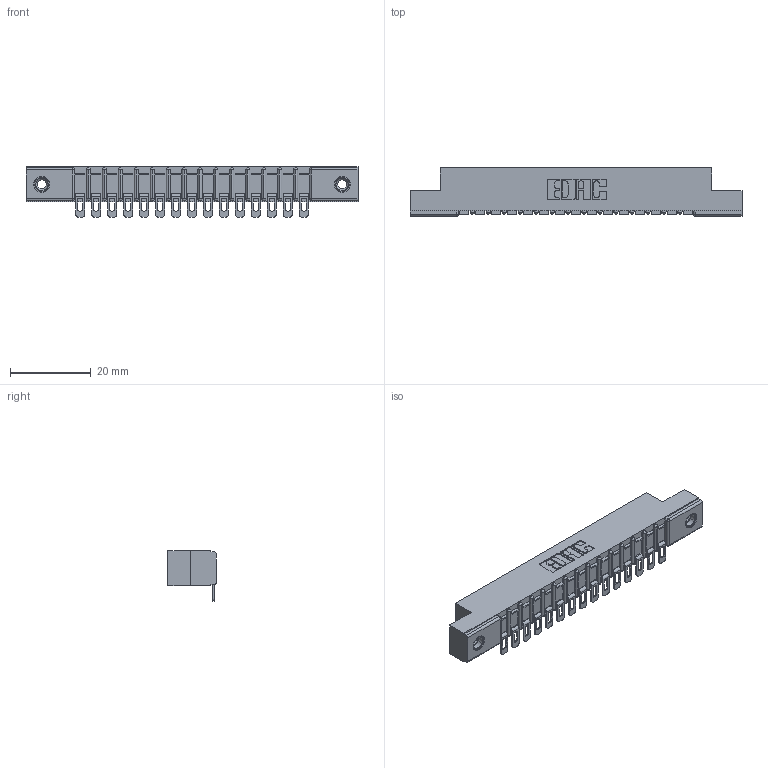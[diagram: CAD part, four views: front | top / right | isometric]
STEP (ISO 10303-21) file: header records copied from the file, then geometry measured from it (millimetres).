
FILE_DESCRIPTION (( 'STEP AP203' ), '1' );
FILE_NAME ('307-015-454-108.STEP', '2020-09-25T18:08:38', ( '' ), ( '' ), 'SwSTEP 2.0', 'SolidWorks 2020', '' );
FILE_SCHEMA (( 'CONFIG_CONTROL_DESIGN' ));
Length unit declared in the file: inch
Products named in the file (4): 307 Part_.156 Dia Mounting Holes; 307-015-454-108; 307-290-002_554; 345-250-001_345-250-003-102
Assembly tree (18 placements, depth 2):
  307-015-454-108
    307 Part_.156 Dia Mounting Holes
    307-290-002_554  x15
    345-250-001_345-250-003-102  x2
Bounding box: 82.45 x 12.01 x 12.52 mm (x, y, z)
Volume: 5438.3 mm3; surface area: 9582.6 mm2
Topology: 18 solids, 18 shells, 1409 faces, 4254 edges, 2784 vertices
Faces by surface type: plane 792, cylinder 569, sphere 32, cone 12, torus 4
Entity records: 18338 total; most frequent: CARTESIAN_POINT 3069, ORIENTED_EDGE 3052, DIRECTION 3010, EDGE_CURVE 1526, VECTOR 1148, LINE 1148, VERTEX_POINT 990, AXIS2_PLACEMENT_3D 931
